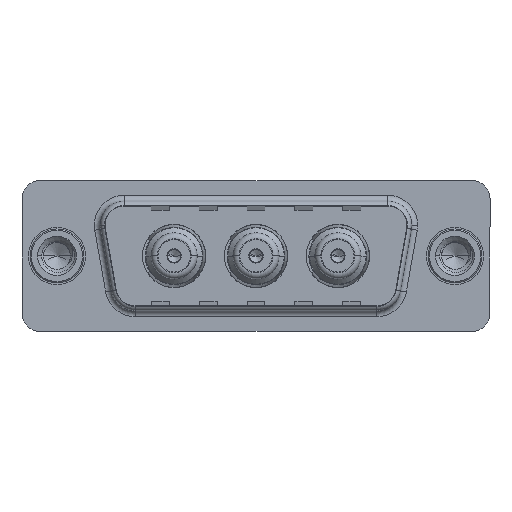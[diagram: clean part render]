
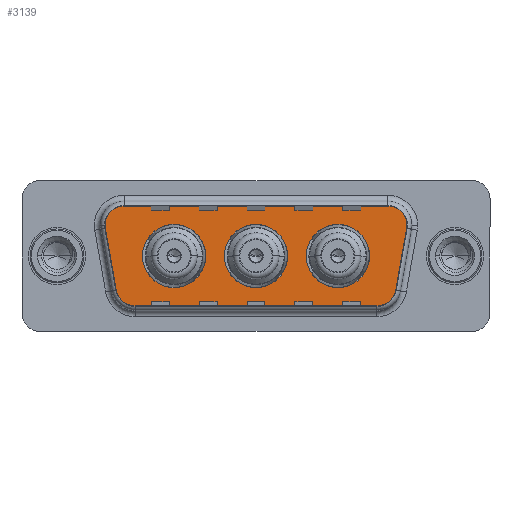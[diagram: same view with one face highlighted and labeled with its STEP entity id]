
A CAD part, top view. The second image highlights one B-rep face of the part: STEP entity #3139.
In plain terms, the highlighted planar face has unit normal (0, 0, 1).
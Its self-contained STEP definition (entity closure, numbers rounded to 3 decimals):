
#280 = CARTESIAN_POINT ( 'NONE',  ( 3.441, 2.553, 0. ) ) ;
#324 = EDGE_CURVE ( 'NONE', #6441, #1304, #7137, .T. ) ;
#349 = DIRECTION ( 'NONE',  ( 0., 0., 1. ) ) ;
#408 = CARTESIAN_POINT ( 'NONE',  ( 5.411, 4.9, 0. ) ) ;
#534 = DIRECTION ( 'NONE',  ( 0., 0., 1. ) ) ;
#584 = VECTOR ( 'NONE', #11427, 1000. ) ;
#817 = AXIS2_PLACEMENT_3D ( 'NONE', #10603, #3287, #11855 ) ;
#895 = CARTESIAN_POINT ( 'NONE',  ( 3.441, 2.553, 0. ) ) ;
#1000 = CIRCLE ( 'NONE', #7858, 2. ) ;
#1108 = AXIS2_PLACEMENT_3D ( 'NONE', #8473, #10011, #8351 ) ;
#1145 = CARTESIAN_POINT ( 'NONE',  ( 9.8, 0., 0. ) ) ;
#1304 = VERTEX_POINT ( 'NONE', #5535 ) ;
#1453 = CARTESIAN_POINT ( 'NONE',  ( 27.889, 2.9, 0. ) ) ;
#1523 = CARTESIAN_POINT ( 'NONE',  ( 7.15, 0., 0. ) ) ;
#1598 = EDGE_LOOP ( 'NONE', ( #8321, #4344 ) ) ;
#2033 = DIRECTION ( 'NONE',  ( 0., 0., 1. ) ) ;
#2063 = CIRCLE ( 'NONE', #14247, 2.65 ) ;
#2095 = AXIS2_PLACEMENT_3D ( 'NONE', #5878, #14909, #13827 ) ;
#2200 = PLANE ( 'NONE',  #2095 ) ;
#2292 = DIRECTION ( 'NONE',  ( 0.174, -0.985, 0. ) ) ;
#2361 = DIRECTION ( 'NONE',  ( 1., 0., 0. ) ) ;
#2435 = VECTOR ( 'NONE', #2971, 1000. ) ;
#2441 = VERTEX_POINT ( 'NONE', #280 ) ;
#2503 = EDGE_CURVE ( 'NONE', #11546, #9197, #6926, .T. ) ;
#2680 = DIRECTION ( 'NONE',  ( -1., 0., 0. ) ) ;
#2750 = CIRCLE ( 'NONE', #12322, 2.65 ) ;
#2859 = FACE_BOUND ( 'NONE', #14516, .T. ) ;
#2946 = DIRECTION ( 'NONE',  ( 0., 0., 1. ) ) ;
#2971 = DIRECTION ( 'NONE',  ( 0.174, 0.985, 0. ) ) ;
#3139 = ADVANCED_FACE ( 'NONE', ( #8597, #2859, #11848, #5369 ), #2200, .T. ) ;
#3228 = CARTESIAN_POINT ( 'NONE',  ( 29.889, 2.9, 0. ) ) ;
#3287 = DIRECTION ( 'NONE',  ( 0., 0., 1. ) ) ;
#3420 = CIRCLE ( 'NONE', #10532, 2.65 ) ;
#3456 = CARTESIAN_POINT ( 'NONE',  ( 12.45, 0., 0. ) ) ;
#3609 = EDGE_CURVE ( 'NONE', #11259, #7284, #12206, .T. ) ;
#3689 = AXIS2_PLACEMENT_3D ( 'NONE', #1453, #10009, #2680 ) ;
#3695 = CIRCLE ( 'NONE', #3689, 2. ) ;
#3831 = LINE ( 'NONE', #408, #584 ) ;
#3867 = DIRECTION ( 'NONE',  ( 0., 0., 1. ) ) ;
#3916 = CARTESIAN_POINT ( 'NONE',  ( 20.85, 0., 0. ) ) ;
#4149 = CARTESIAN_POINT ( 'NONE',  ( 14., 0., 0. ) ) ;
#4344 = ORIENTED_EDGE ( 'NONE', *, *, #12425, .F. ) ;
#4368 = DIRECTION ( 'NONE',  ( 0., 0., 1. ) ) ;
#5120 = VERTEX_POINT ( 'NONE', #4149 ) ;
#5159 = CIRCLE ( 'NONE', #11272, 2.65 ) ;
#5369 = FACE_OUTER_BOUND ( 'NONE', #15153, .T. ) ;
#5490 = CIRCLE ( 'NONE', #1108, 2. ) ;
#5535 = CARTESIAN_POINT ( 'NONE',  ( 27.889, 4.9, 0. ) ) ;
#5648 = DIRECTION ( 'NONE',  ( -1., 0., 0. ) ) ;
#5878 = CARTESIAN_POINT ( 'NONE',  ( 26.866, -2.9, 0. ) ) ;
#6011 = VERTEX_POINT ( 'NONE', #7851 ) ;
#6287 = VERTEX_POINT ( 'NONE', #11083 ) ;
#6315 = ORIENTED_EDGE ( 'NONE', *, *, #15636, .T. ) ;
#6441 = VERTEX_POINT ( 'NONE', #3228 ) ;
#6476 = ORIENTED_EDGE ( 'NONE', *, *, #10210, .T. ) ;
#6482 = CARTESIAN_POINT ( 'NONE',  ( 28.836, -3.247, 0. ) ) ;
#6824 = EDGE_CURVE ( 'NONE', #8316, #2441, #5490, .T. ) ;
#6861 = DIRECTION ( 'NONE',  ( 0., 0., 1. ) ) ;
#6866 = EDGE_CURVE ( 'NONE', #2441, #7779, #11583, .T. ) ;
#6917 = ORIENTED_EDGE ( 'NONE', *, *, #11896, .F. ) ;
#6926 = LINE ( 'NONE', #9374, #13014 ) ;
#6997 = ORIENTED_EDGE ( 'NONE', *, *, #2503, .T. ) ;
#7137 = CIRCLE ( 'NONE', #7938, 2. ) ;
#7284 = VERTEX_POINT ( 'NONE', #7847 ) ;
#7704 = CARTESIAN_POINT ( 'NONE',  ( 23.5, 0., 0. ) ) ;
#7779 = VERTEX_POINT ( 'NONE', #14571 ) ;
#7847 = CARTESIAN_POINT ( 'NONE',  ( 29.859, 2.553, 0. ) ) ;
#7851 = CARTESIAN_POINT ( 'NONE',  ( 26.15, 0., 0. ) ) ;
#7858 = AXIS2_PLACEMENT_3D ( 'NONE', #9370, #2033, #10579 ) ;
#7938 = AXIS2_PLACEMENT_3D ( 'NONE', #12081, #534, #5648 ) ;
#8177 = CARTESIAN_POINT ( 'NONE',  ( 29.859, 2.553, 0. ) ) ;
#8316 = VERTEX_POINT ( 'NONE', #15603 ) ;
#8321 = ORIENTED_EDGE ( 'NONE', *, *, #12168, .F. ) ;
#8351 = DIRECTION ( 'NONE',  ( 1., 0., 0. ) ) ;
#8362 = VECTOR ( 'NONE', #2292, 1000. ) ;
#8366 = VERTEX_POINT ( 'NONE', #3456 ) ;
#8473 = CARTESIAN_POINT ( 'NONE',  ( 5.411, 2.9, 0. ) ) ;
#8597 = FACE_BOUND ( 'NONE', #12551, .T. ) ;
#8917 = DIRECTION ( 'NONE',  ( 1., 0., 0. ) ) ;
#9197 = VERTEX_POINT ( 'NONE', #13558 ) ;
#9370 = CARTESIAN_POINT ( 'NONE',  ( 6.434, -2.9, 0. ) ) ;
#9374 = CARTESIAN_POINT ( 'NONE',  ( 6.434, -4.9, 0. ) ) ;
#9689 = ORIENTED_EDGE ( 'NONE', *, *, #11228, .F. ) ;
#9694 = DIRECTION ( 'NONE',  ( 0., 0., 1. ) ) ;
#9728 = ORIENTED_EDGE ( 'NONE', *, *, #324, .T. ) ;
#10009 = DIRECTION ( 'NONE',  ( 0., 0., 1. ) ) ;
#10011 = DIRECTION ( 'NONE',  ( 0., 0., 1. ) ) ;
#10070 = EDGE_CURVE ( 'NONE', #1304, #8316, #3831, .T. ) ;
#10210 = EDGE_CURVE ( 'NONE', #9197, #11259, #15314, .T. ) ;
#10268 = CARTESIAN_POINT ( 'NONE',  ( 23.5, 0., 0. ) ) ;
#10412 = ORIENTED_EDGE ( 'NONE', *, *, #12259, .F. ) ;
#10532 = AXIS2_PLACEMENT_3D ( 'NONE', #7704, #349, #8917 ) ;
#10579 = DIRECTION ( 'NONE',  ( -1., 0., 0. ) ) ;
#10603 = CARTESIAN_POINT ( 'NONE',  ( 16.65, 0., 0. ) ) ;
#11048 = CIRCLE ( 'NONE', #817, 2.65 ) ;
#11083 = CARTESIAN_POINT ( 'NONE',  ( 19.3, 0., 0. ) ) ;
#11205 = CARTESIAN_POINT ( 'NONE',  ( 16.65, 0., 0. ) ) ;
#11228 = EDGE_CURVE ( 'NONE', #12820, #6011, #3420, .T. ) ;
#11259 = VERTEX_POINT ( 'NONE', #6482 ) ;
#11272 = AXIS2_PLACEMENT_3D ( 'NONE', #10268, #2946, #11497 ) ;
#11427 = DIRECTION ( 'NONE',  ( -1., 0., 0. ) ) ;
#11480 = AXIS2_PLACEMENT_3D ( 'NONE', #1145, #9694, #2361 ) ;
#11497 = DIRECTION ( 'NONE',  ( 1., 0., 0. ) ) ;
#11546 = VERTEX_POINT ( 'NONE', #15573 ) ;
#11583 = LINE ( 'NONE', #895, #8362 ) ;
#11685 = CARTESIAN_POINT ( 'NONE',  ( 26.866, -2.9, 0. ) ) ;
#11848 = FACE_BOUND ( 'NONE', #1598, .T. ) ;
#11855 = DIRECTION ( 'NONE',  ( 1., 0., 0. ) ) ;
#11896 = EDGE_CURVE ( 'NONE', #6011, #12820, #5159, .T. ) ;
#12045 = ORIENTED_EDGE ( 'NONE', *, *, #3609, .T. ) ;
#12081 = CARTESIAN_POINT ( 'NONE',  ( 27.889, 2.9, 0. ) ) ;
#12168 = EDGE_CURVE ( 'NONE', #8366, #12853, #2063, .T. ) ;
#12206 = LINE ( 'NONE', #8177, #2435 ) ;
#12259 = EDGE_CURVE ( 'NONE', #6287, #5120, #11048, .T. ) ;
#12322 = AXIS2_PLACEMENT_3D ( 'NONE', #11205, #3867, #12437 ) ;
#12425 = EDGE_CURVE ( 'NONE', #12853, #8366, #15249, .T. ) ;
#12437 = DIRECTION ( 'NONE',  ( 1., 0., 0. ) ) ;
#12551 = EDGE_LOOP ( 'NONE', ( #10412, #13528 ) ) ;
#12820 = VERTEX_POINT ( 'NONE', #3916 ) ;
#12853 = VERTEX_POINT ( 'NONE', #1523 ) ;
#12932 = DIRECTION ( 'NONE',  ( 1., 0., 0. ) ) ;
#13011 = DIRECTION ( 'NONE',  ( 1., 0., 0. ) ) ;
#13014 = VECTOR ( 'NONE', #13011, 1000. ) ;
#13457 = EDGE_CURVE ( 'NONE', #7284, #6441, #3695, .T. ) ;
#13475 = ORIENTED_EDGE ( 'NONE', *, *, #10070, .T. ) ;
#13528 = ORIENTED_EDGE ( 'NONE', *, *, #14676, .F. ) ;
#13558 = CARTESIAN_POINT ( 'NONE',  ( 26.866, -4.9, 0. ) ) ;
#13715 = ORIENTED_EDGE ( 'NONE', *, *, #13457, .T. ) ;
#13827 = DIRECTION ( 'NONE',  ( 1., 0., 0. ) ) ;
#13864 = AXIS2_PLACEMENT_3D ( 'NONE', #11685, #4368, #12932 ) ;
#14155 = CARTESIAN_POINT ( 'NONE',  ( 9.8, 0., 0. ) ) ;
#14247 = AXIS2_PLACEMENT_3D ( 'NONE', #14155, #6861, #15375 ) ;
#14417 = ORIENTED_EDGE ( 'NONE', *, *, #6866, .T. ) ;
#14516 = EDGE_LOOP ( 'NONE', ( #6917, #9689 ) ) ;
#14571 = CARTESIAN_POINT ( 'NONE',  ( 4.464, -3.247, 0. ) ) ;
#14676 = EDGE_CURVE ( 'NONE', #5120, #6287, #2750, .T. ) ;
#14685 = ORIENTED_EDGE ( 'NONE', *, *, #6824, .T. ) ;
#14909 = DIRECTION ( 'NONE',  ( 0., 0., 1. ) ) ;
#15153 = EDGE_LOOP ( 'NONE', ( #6476, #12045, #13715, #9728, #13475, #14685, #14417, #6315, #6997 ) ) ;
#15249 = CIRCLE ( 'NONE', #11480, 2.65 ) ;
#15314 = CIRCLE ( 'NONE', #13864, 2. ) ;
#15375 = DIRECTION ( 'NONE',  ( 1., 0., 0. ) ) ;
#15573 = CARTESIAN_POINT ( 'NONE',  ( 6.434, -4.9, 0. ) ) ;
#15603 = CARTESIAN_POINT ( 'NONE',  ( 5.411, 4.9, 0. ) ) ;
#15636 = EDGE_CURVE ( 'NONE', #7779, #11546, #1000, .T. ) ;
